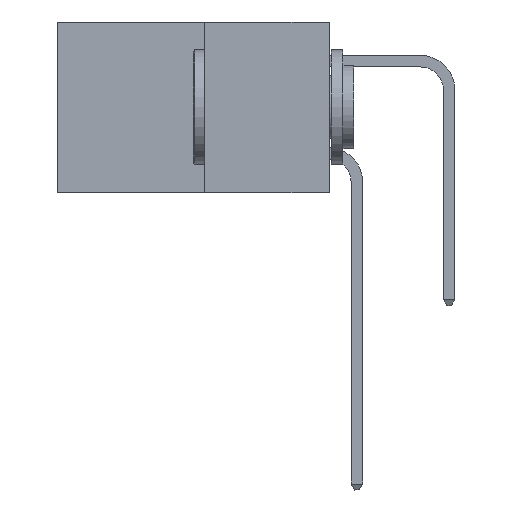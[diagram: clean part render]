
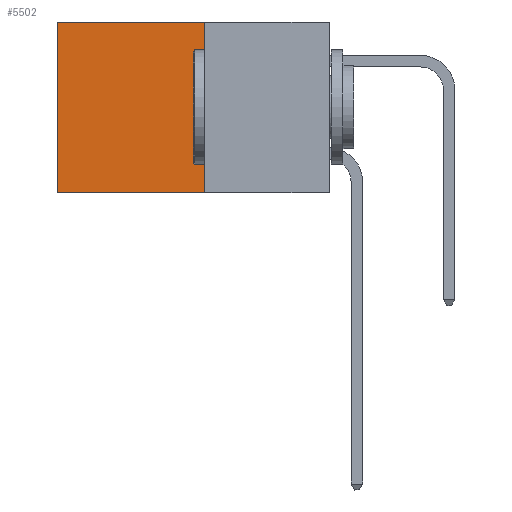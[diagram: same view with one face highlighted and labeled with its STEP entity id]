
A CAD part, left-side view. The second image highlights one B-rep face of the part: STEP entity #5502.
In plain terms, the highlighted planar face has unit normal (-1, 0, 0).
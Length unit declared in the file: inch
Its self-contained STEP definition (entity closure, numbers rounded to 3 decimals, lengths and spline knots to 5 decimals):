
#543 = EDGE_LOOP ( 'NONE', ( #654, #9910, #28157, #7273 ) ) ;
#654 = ORIENTED_EDGE ( 'NONE', *, *, #33942, .T. ) ;
#777 = VECTOR ( 'NONE', #11656, 39.37008 ) ;
#1992 = VERTEX_POINT ( 'NONE', #18608 ) ;
#2855 = CARTESIAN_POINT ( 'NONE',  ( 0.277, 0.59, -0.37 ) ) ;
#2925 = AXIS2_PLACEMENT_3D ( 'NONE', #4107, #4059, #3979 ) ;
#3979 = DIRECTION ( 'NONE',  ( 0., 0., -1. ) ) ;
#4059 = DIRECTION ( 'NONE',  ( 1., 0., 0. ) ) ;
#4107 = CARTESIAN_POINT ( 'NONE',  ( 0.277, 0.27, -0.37 ) ) ;
#4306 = PLANE ( 'NONE',  #2925 ) ;
#5338 = CARTESIAN_POINT ( 'NONE',  ( 0.277, 0.27, 0. ) ) ;
#5502 = ADVANCED_FACE ( 'NONE', ( #24112 ), #4306, .F. ) ;
#6182 = CARTESIAN_POINT ( 'NONE',  ( 0.277, 0.27, -0.37 ) ) ;
#7273 = ORIENTED_EDGE ( 'NONE', *, *, #13487, .T. ) ;
#7286 = VECTOR ( 'NONE', #8198, 39.37008 ) ;
#8198 = DIRECTION ( 'NONE',  ( 0., 0., -1. ) ) ;
#9910 = ORIENTED_EDGE ( 'NONE', *, *, #19294, .F. ) ;
#10520 = CARTESIAN_POINT ( 'NONE',  ( 0.277, 0.59, 0. ) ) ;
#11656 = DIRECTION ( 'NONE',  ( 0., 0., -1. ) ) ;
#13369 = VERTEX_POINT ( 'NONE', #10520 ) ;
#13487 = EDGE_CURVE ( 'NONE', #1992, #13369, #26052, .T. ) ;
#14265 = VERTEX_POINT ( 'NONE', #2855 ) ;
#15423 = CARTESIAN_POINT ( 'NONE',  ( 0.277, 0.27, -0.37 ) ) ;
#16423 = CARTESIAN_POINT ( 'NONE',  ( 0.277, 0.27, -0.37 ) ) ;
#17868 = VECTOR ( 'NONE', #30115, 39.37008 ) ;
#18194 = DIRECTION ( 'NONE',  ( 0., 1., 0. ) ) ;
#18608 = CARTESIAN_POINT ( 'NONE',  ( 0.277, 0.27, 0. ) ) ;
#19294 = EDGE_CURVE ( 'NONE', #30083, #14265, #35522, .T. ) ;
#24112 = FACE_OUTER_BOUND ( 'NONE', #543, .T. ) ;
#26052 = LINE ( 'NONE', #5338, #17868 ) ;
#26754 = VECTOR ( 'NONE', #18194, 39.37008 ) ;
#28046 = CARTESIAN_POINT ( 'NONE',  ( 0.277, 0.59, -0.37 ) ) ;
#28157 = ORIENTED_EDGE ( 'NONE', *, *, #29905, .F. ) ;
#28409 = LINE ( 'NONE', #28046, #777 ) ;
#29905 = EDGE_CURVE ( 'NONE', #1992, #30083, #35487, .T. ) ;
#30083 = VERTEX_POINT ( 'NONE', #6182 ) ;
#30115 = DIRECTION ( 'NONE',  ( 0., 1., 0. ) ) ;
#33942 = EDGE_CURVE ( 'NONE', #13369, #14265, #28409, .T. ) ;
#35487 = LINE ( 'NONE', #16423, #7286 ) ;
#35522 = LINE ( 'NONE', #15423, #26754 ) ;
